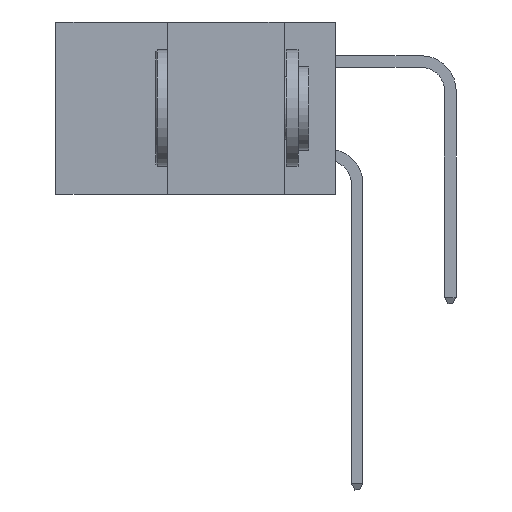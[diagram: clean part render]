
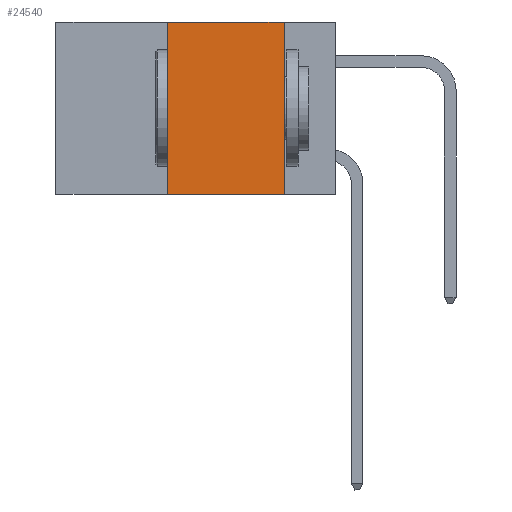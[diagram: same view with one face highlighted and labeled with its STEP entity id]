
A CAD part, left-side view. The second image highlights one B-rep face of the part: STEP entity #24540.
In plain terms, the highlighted planar face has unit normal (-1, 0, 0).
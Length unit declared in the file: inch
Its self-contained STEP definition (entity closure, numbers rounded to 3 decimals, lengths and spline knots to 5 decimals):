
#286 = DIRECTION ( 'NONE',  ( 0., 0., 1. ) ) ;
#538 = VERTEX_POINT ( 'NONE', #26648 ) ;
#804 = CARTESIAN_POINT ( 'NONE',  ( 0., 0.6, -0.37 ) ) ;
#1457 = LINE ( 'NONE', #2609, #8186 ) ;
#1854 = ORIENTED_EDGE ( 'NONE', *, *, #27174, .T. ) ;
#2609 = CARTESIAN_POINT ( 'NONE',  ( 0., 0.36, 0. ) ) ;
#4166 = VECTOR ( 'NONE', #6134, 39.37008 ) ;
#4882 = DIRECTION ( 'NONE',  ( 0., 0., -1. ) ) ;
#6134 = DIRECTION ( 'NONE',  ( 0., 0., -1. ) ) ;
#7427 = FACE_OUTER_BOUND ( 'NONE', #9697, .T. ) ;
#7843 = AXIS2_PLACEMENT_3D ( 'NONE', #13511, #17904, #4882 ) ;
#8186 = VECTOR ( 'NONE', #286, 39.37008 ) ;
#9454 = CARTESIAN_POINT ( 'NONE',  ( 0., 0.36, 0. ) ) ;
#9697 = EDGE_LOOP ( 'NONE', ( #17510, #20243, #14882, #1854 ) ) ;
#9826 = DIRECTION ( 'NONE',  ( 0., -1., 0. ) ) ;
#10349 = VERTEX_POINT ( 'NONE', #24296 ) ;
#10413 = VERTEX_POINT ( 'NONE', #9454 ) ;
#12068 = VERTEX_POINT ( 'NONE', #14631 ) ;
#12081 = VECTOR ( 'NONE', #25356, 39.37008 ) ;
#13511 = CARTESIAN_POINT ( 'NONE',  ( 0., 0.6, 0. ) ) ;
#14479 = VECTOR ( 'NONE', #9826, 39.37008 ) ;
#14631 = CARTESIAN_POINT ( 'NONE',  ( 0., 0.11, -0.37 ) ) ;
#14882 = ORIENTED_EDGE ( 'NONE', *, *, #25939, .F. ) ;
#15727 = PLANE ( 'NONE',  #7843 ) ;
#17003 = EDGE_CURVE ( 'NONE', #10413, #538, #17180, .T. ) ;
#17180 = LINE ( 'NONE', #27506, #12081 ) ;
#17510 = ORIENTED_EDGE ( 'NONE', *, *, #19628, .F. ) ;
#17904 = DIRECTION ( 'NONE',  ( 1., 0., 0. ) ) ;
#19112 = CARTESIAN_POINT ( 'NONE',  ( 0., 0.11, 0. ) ) ;
#19628 = EDGE_CURVE ( 'NONE', #538, #12068, #27214, .T. ) ;
#20243 = ORIENTED_EDGE ( 'NONE', *, *, #17003, .F. ) ;
#24296 = CARTESIAN_POINT ( 'NONE',  ( 0., 0.36, -0.37 ) ) ;
#24540 = ADVANCED_FACE ( 'NONE', ( #7427 ), #15727, .F. ) ;
#25356 = DIRECTION ( 'NONE',  ( 0., -1., 0. ) ) ;
#25939 = EDGE_CURVE ( 'NONE', #10349, #10413, #1457, .T. ) ;
#26623 = LINE ( 'NONE', #804, #14479 ) ;
#26648 = CARTESIAN_POINT ( 'NONE',  ( 0., 0.11, 0. ) ) ;
#27174 = EDGE_CURVE ( 'NONE', #10349, #12068, #26623, .T. ) ;
#27214 = LINE ( 'NONE', #19112, #4166 ) ;
#27506 = CARTESIAN_POINT ( 'NONE',  ( 0., 0.6, 0. ) ) ;
